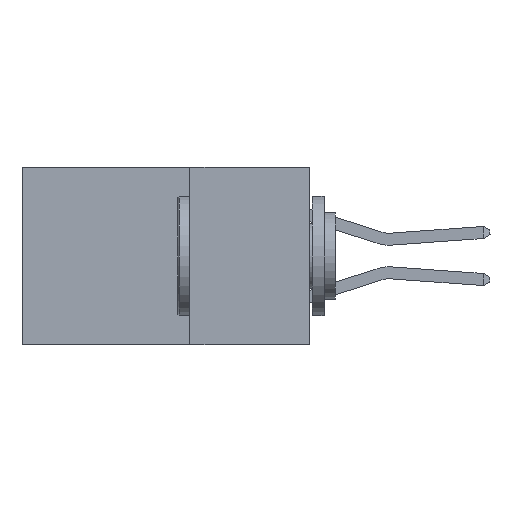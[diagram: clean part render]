
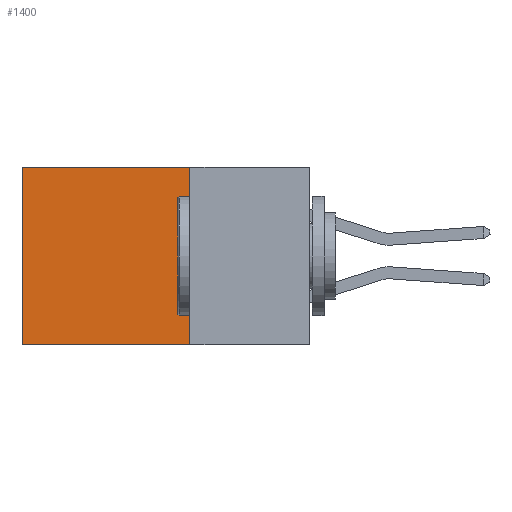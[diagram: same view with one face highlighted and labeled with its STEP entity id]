
A CAD part, left-side view. The second image highlights one B-rep face of the part: STEP entity #1400.
In plain terms, the highlighted planar face has unit normal (-1, 0, 0).
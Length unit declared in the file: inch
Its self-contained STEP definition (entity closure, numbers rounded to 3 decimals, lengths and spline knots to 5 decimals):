
#543 = CARTESIAN_POINT ( 'NONE',  ( 0.2615, 0.25, -0.37 ) ) ;
#832 = CARTESIAN_POINT ( 'NONE',  ( 0.2615, 0.25, 0. ) ) ;
#1078 = LINE ( 'NONE', #24953, #13201 ) ;
#1400 = ADVANCED_FACE ( 'NONE', ( #18037 ), #4525, .F. ) ;
#1978 = VERTEX_POINT ( 'NONE', #14694 ) ;
#2040 = ORIENTED_EDGE ( 'NONE', *, *, #9510, .T. ) ;
#2207 = CARTESIAN_POINT ( 'NONE',  ( 0.2615, 0.25, -0.37 ) ) ;
#2864 = DIRECTION ( 'NONE',  ( 0., 0., -1. ) ) ;
#3174 = EDGE_CURVE ( 'NONE', #7241, #1978, #1078, .T. ) ;
#4525 = PLANE ( 'NONE',  #6984 ) ;
#5527 = CARTESIAN_POINT ( 'NONE',  ( 0.2615, 0.6, -0.37 ) ) ;
#6261 = EDGE_CURVE ( 'NONE', #7241, #23838, #17416, .T. ) ;
#6984 = AXIS2_PLACEMENT_3D ( 'NONE', #543, #13961, #2864 ) ;
#7241 = VERTEX_POINT ( 'NONE', #832 ) ;
#7442 = DIRECTION ( 'NONE',  ( 0., 0., -1. ) ) ;
#7613 = DIRECTION ( 'NONE',  ( 0., 1., 0. ) ) ;
#8995 = LINE ( 'NONE', #5527, #23300 ) ;
#9280 = EDGE_CURVE ( 'NONE', #1978, #15079, #13701, .T. ) ;
#9490 = EDGE_LOOP ( 'NONE', ( #2040, #24786, #23239, #16529 ) ) ;
#9510 = EDGE_CURVE ( 'NONE', #23838, #15079, #8995, .T. ) ;
#11300 = DIRECTION ( 'NONE',  ( 0., 0., -1. ) ) ;
#11334 = CARTESIAN_POINT ( 'NONE',  ( 0.2615, 0.6, 0. ) ) ;
#13201 = VECTOR ( 'NONE', #11300, 39.37008 ) ;
#13640 = CARTESIAN_POINT ( 'NONE',  ( 0.2615, 0.6, -0.37 ) ) ;
#13701 = LINE ( 'NONE', #2207, #18803 ) ;
#13961 = DIRECTION ( 'NONE',  ( 1., 0., 0. ) ) ;
#14694 = CARTESIAN_POINT ( 'NONE',  ( 0.2615, 0.25, -0.37 ) ) ;
#15079 = VERTEX_POINT ( 'NONE', #13640 ) ;
#16529 = ORIENTED_EDGE ( 'NONE', *, *, #6261, .T. ) ;
#17416 = LINE ( 'NONE', #23294, #19990 ) ;
#18037 = FACE_OUTER_BOUND ( 'NONE', #9490, .T. ) ;
#18803 = VECTOR ( 'NONE', #21736, 39.37008 ) ;
#19990 = VECTOR ( 'NONE', #7613, 39.37008 ) ;
#21736 = DIRECTION ( 'NONE',  ( 0., 1., 0. ) ) ;
#23239 = ORIENTED_EDGE ( 'NONE', *, *, #3174, .F. ) ;
#23294 = CARTESIAN_POINT ( 'NONE',  ( 0.2615, 0.25, 0. ) ) ;
#23300 = VECTOR ( 'NONE', #7442, 39.37008 ) ;
#23838 = VERTEX_POINT ( 'NONE', #11334 ) ;
#24786 = ORIENTED_EDGE ( 'NONE', *, *, #9280, .F. ) ;
#24953 = CARTESIAN_POINT ( 'NONE',  ( 0.2615, 0.25, -0.37 ) ) ;
